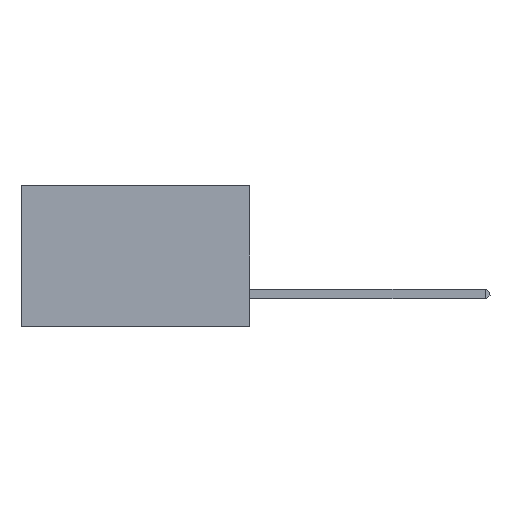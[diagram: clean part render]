
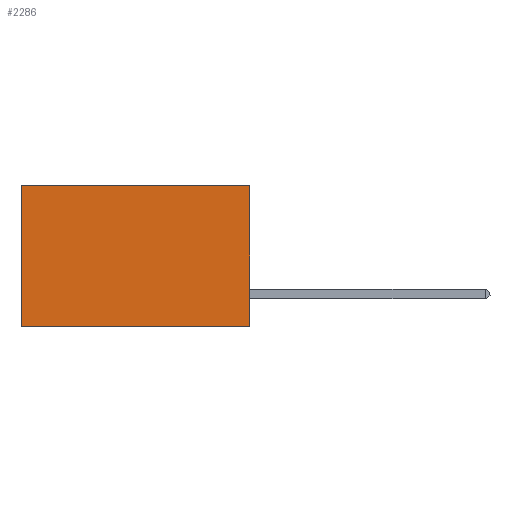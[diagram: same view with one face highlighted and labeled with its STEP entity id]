
A CAD part, left-side view. The second image highlights one B-rep face of the part: STEP entity #2286.
In plain terms, the highlighted planar face has unit normal (-1, 0, 0).
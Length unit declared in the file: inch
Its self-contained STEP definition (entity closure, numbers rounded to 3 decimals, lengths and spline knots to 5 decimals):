
#165 = CARTESIAN_POINT ( 'NONE',  ( 0.2875, 0., 0. ) ) ;
#1329 = CARTESIAN_POINT ( 'NONE',  ( 0.2875, 0.6, 0. ) ) ;
#1672 = VERTEX_POINT ( 'NONE', #8522 ) ;
#1979 = LINE ( 'NONE', #1329, #3516 ) ;
#2235 = CARTESIAN_POINT ( 'NONE',  ( 0.2875, 0., -0.37 ) ) ;
#2286 = ADVANCED_FACE ( 'NONE', ( #11588 ), #11469, .F. ) ;
#2466 = ORIENTED_EDGE ( 'NONE', *, *, #6809, .T. ) ;
#2612 = LINE ( 'NONE', #165, #12529 ) ;
#2707 = EDGE_CURVE ( 'NONE', #10637, #1672, #2612, .T. ) ;
#2892 = VERTEX_POINT ( 'NONE', #6437 ) ;
#3088 = DIRECTION ( 'NONE',  ( 0., 0., -1. ) ) ;
#3492 = VERTEX_POINT ( 'NONE', #3892 ) ;
#3516 = VECTOR ( 'NONE', #8242, 39.37008 ) ;
#3892 = CARTESIAN_POINT ( 'NONE',  ( 0.2875, 0.6, -0.37 ) ) ;
#5459 = DIRECTION ( 'NONE',  ( 0., 1., 0. ) ) ;
#5774 = VECTOR ( 'NONE', #5459, 39.37008 ) ;
#6395 = LINE ( 'NONE', #10383, #5774 ) ;
#6437 = CARTESIAN_POINT ( 'NONE',  ( 0.2875, 0.6, 0. ) ) ;
#6809 = EDGE_CURVE ( 'NONE', #10637, #2892, #6395, .T. ) ;
#8242 = DIRECTION ( 'NONE',  ( 0., 0., -1. ) ) ;
#8274 = CARTESIAN_POINT ( 'NONE',  ( 0.2875, 0., 0. ) ) ;
#8344 = DIRECTION ( 'NONE',  ( 0., 0., -1. ) ) ;
#8522 = CARTESIAN_POINT ( 'NONE',  ( 0.2875, 0., -0.37 ) ) ;
#9396 = EDGE_CURVE ( 'NONE', #2892, #3492, #1979, .T. ) ;
#9656 = EDGE_CURVE ( 'NONE', #1672, #3492, #12029, .T. ) ;
#9695 = VECTOR ( 'NONE', #12672, 39.37008 ) ;
#10383 = CARTESIAN_POINT ( 'NONE',  ( 0.2875, 0., 0. ) ) ;
#10637 = VERTEX_POINT ( 'NONE', #8274 ) ;
#11385 = CARTESIAN_POINT ( 'NONE',  ( 0.2875, 0., 0. ) ) ;
#11469 = PLANE ( 'NONE',  #11589 ) ;
#11481 = EDGE_LOOP ( 'NONE', ( #11700, #12498, #12189, #2466 ) ) ;
#11588 = FACE_OUTER_BOUND ( 'NONE', #11481, .T. ) ;
#11589 = AXIS2_PLACEMENT_3D ( 'NONE', #11385, #12323, #8344 ) ;
#11700 = ORIENTED_EDGE ( 'NONE', *, *, #9396, .T. ) ;
#12029 = LINE ( 'NONE', #2235, #9695 ) ;
#12189 = ORIENTED_EDGE ( 'NONE', *, *, #2707, .F. ) ;
#12323 = DIRECTION ( 'NONE',  ( 1., 0., 0. ) ) ;
#12498 = ORIENTED_EDGE ( 'NONE', *, *, #9656, .F. ) ;
#12529 = VECTOR ( 'NONE', #3088, 39.37008 ) ;
#12672 = DIRECTION ( 'NONE',  ( 0., 1., 0. ) ) ;
